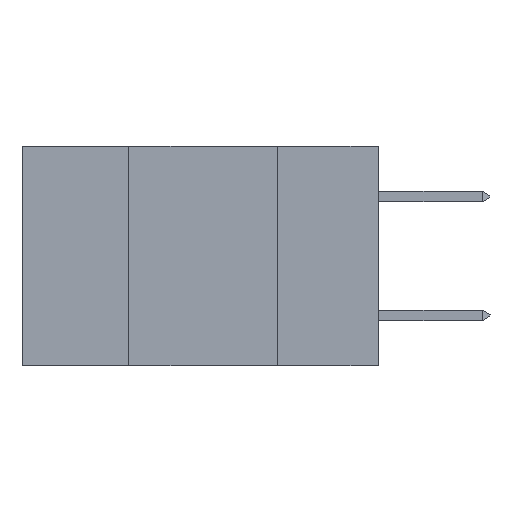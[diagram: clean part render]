
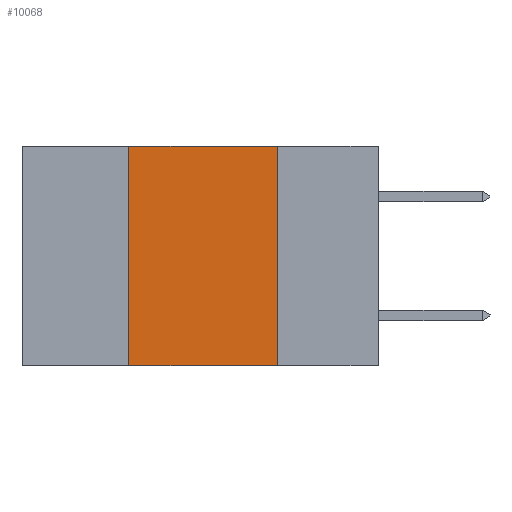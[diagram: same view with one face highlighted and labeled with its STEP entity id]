
A CAD part, left-side view. The second image highlights one B-rep face of the part: STEP entity #10068.
In plain terms, the highlighted planar face has unit normal (-1, 0, 0).
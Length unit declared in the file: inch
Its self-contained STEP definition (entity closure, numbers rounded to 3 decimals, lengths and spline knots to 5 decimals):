
#93 = DIRECTION ( 'NONE',  ( 0., 0., -1. ) ) ;
#1323 = CARTESIAN_POINT ( 'NONE',  ( 0., 0.42, -0.37 ) ) ;
#5276 = EDGE_LOOP ( 'NONE', ( #30430, #18224, #9808, #11948 ) ) ;
#5527 = VERTEX_POINT ( 'NONE', #1323 ) ;
#5786 = VECTOR ( 'NONE', #22692, 39.37008 ) ;
#6235 = LINE ( 'NONE', #20025, #24593 ) ;
#7224 = LINE ( 'NONE', #10990, #31269 ) ;
#9750 = VERTEX_POINT ( 'NONE', #27236 ) ;
#9808 = ORIENTED_EDGE ( 'NONE', *, *, #21038, .F. ) ;
#10068 = ADVANCED_FACE ( 'NONE', ( #10442 ), #23603, .F. ) ;
#10442 = FACE_OUTER_BOUND ( 'NONE', #5276, .T. ) ;
#10990 = CARTESIAN_POINT ( 'NONE',  ( 0., 0.42, 0. ) ) ;
#11098 = DIRECTION ( 'NONE',  ( 0., 0., 1. ) ) ;
#11511 = CARTESIAN_POINT ( 'NONE',  ( 0., 0.17, 0. ) ) ;
#11948 = ORIENTED_EDGE ( 'NONE', *, *, #17659, .T. ) ;
#12529 = LINE ( 'NONE', #12833, #5786 ) ;
#12833 = CARTESIAN_POINT ( 'NONE',  ( 0., 0.6, 0. ) ) ;
#13465 = VERTEX_POINT ( 'NONE', #11511 ) ;
#13725 = CARTESIAN_POINT ( 'NONE',  ( 0., 0.6, -0.37 ) ) ;
#13763 = DIRECTION ( 'NONE',  ( 1., 0., 0. ) ) ;
#17659 = EDGE_CURVE ( 'NONE', #5527, #9750, #18920, .T. ) ;
#18224 = ORIENTED_EDGE ( 'NONE', *, *, #24273, .F. ) ;
#18834 = CARTESIAN_POINT ( 'NONE',  ( 0., 0.42, 0. ) ) ;
#18920 = LINE ( 'NONE', #13725, #25474 ) ;
#19364 = EDGE_CURVE ( 'NONE', #13465, #9750, #6235, .T. ) ;
#20025 = CARTESIAN_POINT ( 'NONE',  ( 0., 0.17, 0. ) ) ;
#21038 = EDGE_CURVE ( 'NONE', #5527, #26559, #7224, .T. ) ;
#22692 = DIRECTION ( 'NONE',  ( 0., -1., 0. ) ) ;
#23561 = AXIS2_PLACEMENT_3D ( 'NONE', #28465, #13763, #30974 ) ;
#23603 = PLANE ( 'NONE',  #23561 ) ;
#24273 = EDGE_CURVE ( 'NONE', #26559, #13465, #12529, .T. ) ;
#24593 = VECTOR ( 'NONE', #93, 39.37008 ) ;
#25474 = VECTOR ( 'NONE', #30933, 39.37008 ) ;
#26559 = VERTEX_POINT ( 'NONE', #18834 ) ;
#27236 = CARTESIAN_POINT ( 'NONE',  ( 0., 0.17, -0.37 ) ) ;
#28465 = CARTESIAN_POINT ( 'NONE',  ( 0., 0.6, 0. ) ) ;
#30430 = ORIENTED_EDGE ( 'NONE', *, *, #19364, .F. ) ;
#30933 = DIRECTION ( 'NONE',  ( 0., -1., 0. ) ) ;
#30974 = DIRECTION ( 'NONE',  ( 0., 0., -1. ) ) ;
#31269 = VECTOR ( 'NONE', #11098, 39.37008 ) ;
